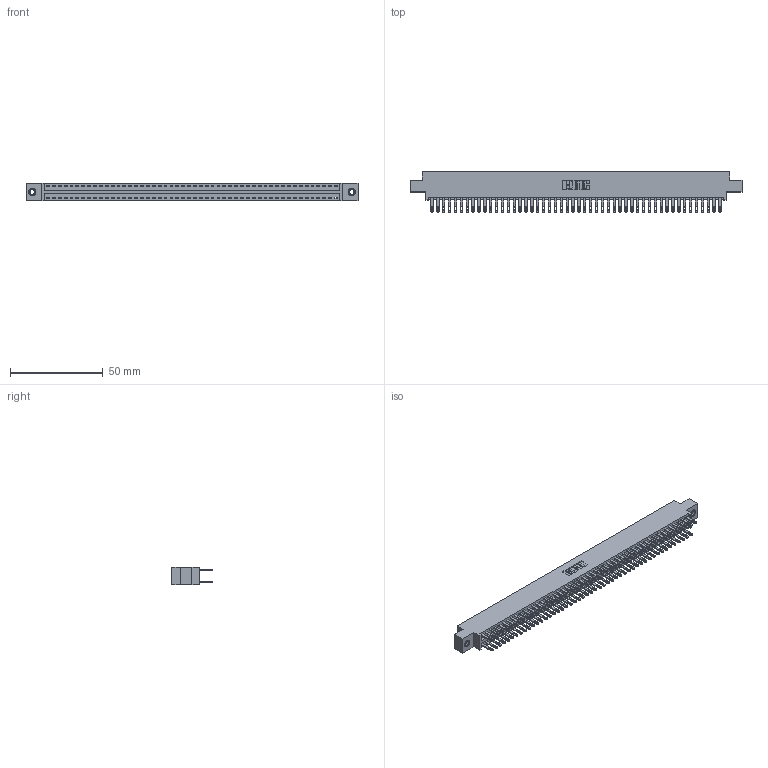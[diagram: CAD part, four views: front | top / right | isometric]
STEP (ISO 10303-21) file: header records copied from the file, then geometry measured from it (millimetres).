
FILE_DESCRIPTION (( 'STEP AP203' ), '1' );
FILE_NAME ('896-100-500-807.STEP', '2021-07-28T03:48:48', ( '' ), ( '' ), 'SwSTEP 2.0', 'SolidWorks 2020', '' );
FILE_SCHEMA (( 'CONFIG_CONTROL_DESIGN' ));
Length unit declared in the file: inch
Products named in the file (4): 345-250-001_345-250-005-103; 896-100-500-807; 345-292-001_345-293-100; 846 Part_0.170 Offset - 0.156 Dia-TI
Assembly tree (102 placements, depth 2):
  896-100-500-807
    846 Part_0.170 Offset - 0.156 Dia-TI
    345-292-001_345-293-100  x99
    345-250-001_345-250-005-103  x2
Bounding box: 179.32 x 21.84 x 9.4 mm (x, y, z)
Volume: 17673.9 mm3; surface area: 25617.3 mm2
Topology: 102 solids, 102 shells, 4944 faces, 15051 edges, 10026 vertices
Faces by surface type: plane 2988, cylinder 1940, cone 12, torus 4
Entity records: 32770 total; most frequent: CARTESIAN_POINT 5378, ORIENTED_EDGE 5306, DIRECTION 4817, EDGE_CURVE 2653, VECTOR 2297, LINE 2297, VERTEX_POINT 1764, AXIS2_PLACEMENT_3D 1260
